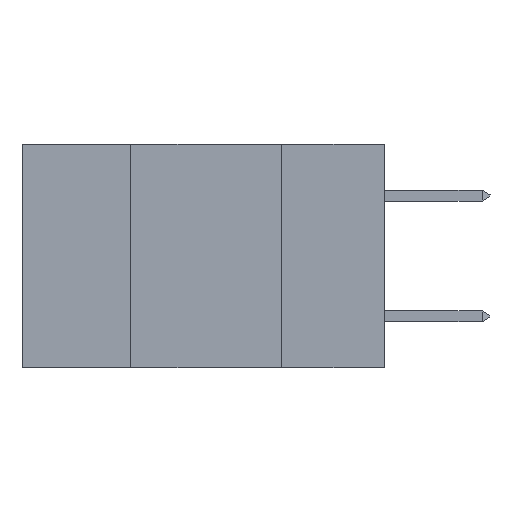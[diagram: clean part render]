
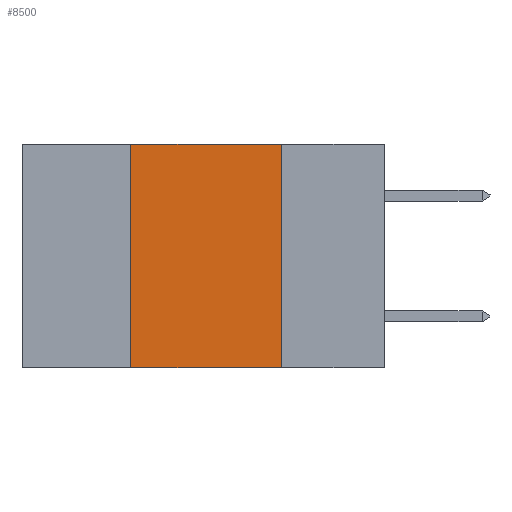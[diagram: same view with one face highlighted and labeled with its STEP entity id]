
A CAD part, left-side view. The second image highlights one B-rep face of the part: STEP entity #8500.
In plain terms, the highlighted planar face has unit normal (-1, 0, 0).
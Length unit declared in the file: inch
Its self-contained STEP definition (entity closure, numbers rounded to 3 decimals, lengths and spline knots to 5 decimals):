
#18 = VECTOR ( 'NONE', #8288, 39.37008 ) ;
#144 = DIRECTION ( 'NONE',  ( 1., 0., 0. ) ) ;
#648 = LINE ( 'NONE', #15537, #18 ) ;
#699 = VERTEX_POINT ( 'NONE', #1071 ) ;
#914 = LINE ( 'NONE', #983, #13576 ) ;
#983 = CARTESIAN_POINT ( 'NONE',  ( 0., 0.6, 0. ) ) ;
#1071 = CARTESIAN_POINT ( 'NONE',  ( 0., 0.17, -0.37 ) ) ;
#2285 = ORIENTED_EDGE ( 'NONE', *, *, #4701, .T. ) ;
#2975 = ORIENTED_EDGE ( 'NONE', *, *, #14801, .F. ) ;
#3419 = CARTESIAN_POINT ( 'NONE',  ( 0., 0.42, 0. ) ) ;
#4701 = EDGE_CURVE ( 'NONE', #10569, #699, #6772, .T. ) ;
#4963 = PLANE ( 'NONE',  #12099 ) ;
#5388 = EDGE_LOOP ( 'NONE', ( #2975, #14465, #7556, #2285 ) ) ;
#5438 = VECTOR ( 'NONE', #14120, 39.37008 ) ;
#6095 = EDGE_CURVE ( 'NONE', #11588, #13896, #914, .T. ) ;
#6604 = DIRECTION ( 'NONE',  ( 0., 0., -1. ) ) ;
#6772 = LINE ( 'NONE', #8890, #5438 ) ;
#7337 = DIRECTION ( 'NONE',  ( 0., 0., -1. ) ) ;
#7556 = ORIENTED_EDGE ( 'NONE', *, *, #11595, .F. ) ;
#8288 = DIRECTION ( 'NONE',  ( 0., 0., 1. ) ) ;
#8500 = ADVANCED_FACE ( 'NONE', ( #8544 ), #4963, .F. ) ;
#8544 = FACE_OUTER_BOUND ( 'NONE', #5388, .T. ) ;
#8871 = CARTESIAN_POINT ( 'NONE',  ( 0., 0.17, 0. ) ) ;
#8890 = CARTESIAN_POINT ( 'NONE',  ( 0., 0.6, -0.37 ) ) ;
#9334 = LINE ( 'NONE', #8871, #15699 ) ;
#10569 = VERTEX_POINT ( 'NONE', #13518 ) ;
#11588 = VERTEX_POINT ( 'NONE', #3419 ) ;
#11595 = EDGE_CURVE ( 'NONE', #10569, #11588, #648, .T. ) ;
#12099 = AXIS2_PLACEMENT_3D ( 'NONE', #14982, #144, #7337 ) ;
#13518 = CARTESIAN_POINT ( 'NONE',  ( 0., 0.42, -0.37 ) ) ;
#13576 = VECTOR ( 'NONE', #15560, 39.37008 ) ;
#13896 = VERTEX_POINT ( 'NONE', #15507 ) ;
#14120 = DIRECTION ( 'NONE',  ( 0., -1., 0. ) ) ;
#14465 = ORIENTED_EDGE ( 'NONE', *, *, #6095, .F. ) ;
#14801 = EDGE_CURVE ( 'NONE', #13896, #699, #9334, .T. ) ;
#14982 = CARTESIAN_POINT ( 'NONE',  ( 0., 0.6, 0. ) ) ;
#15507 = CARTESIAN_POINT ( 'NONE',  ( 0., 0.17, 0. ) ) ;
#15537 = CARTESIAN_POINT ( 'NONE',  ( 0., 0.42, 0. ) ) ;
#15560 = DIRECTION ( 'NONE',  ( 0., -1., 0. ) ) ;
#15699 = VECTOR ( 'NONE', #6604, 39.37008 ) ;
